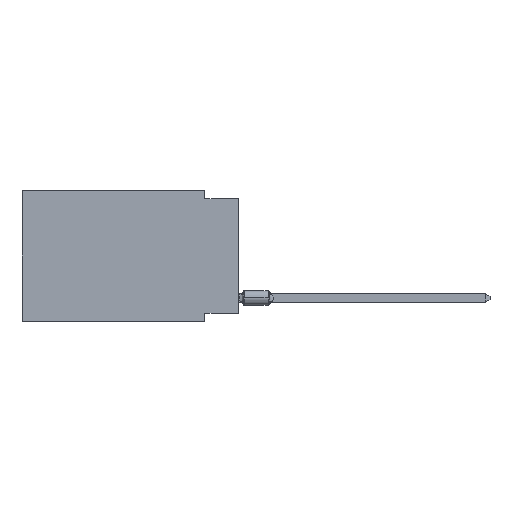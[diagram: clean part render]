
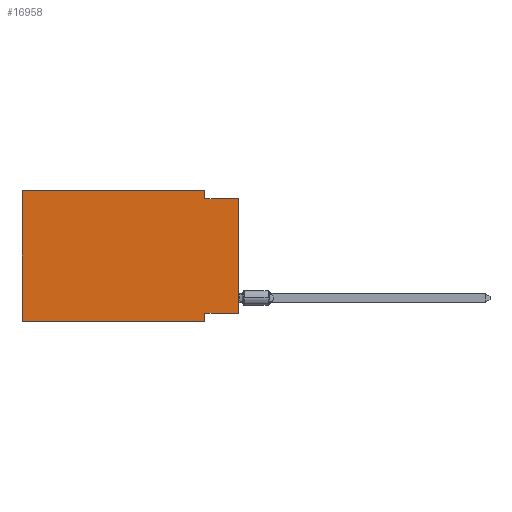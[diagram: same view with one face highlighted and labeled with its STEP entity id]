
A CAD part, left-side view. The second image highlights one B-rep face of the part: STEP entity #16958.
In plain terms, the highlighted planar face has unit normal (-1, 0, 0).
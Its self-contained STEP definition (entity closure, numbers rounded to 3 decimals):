
#176 = LINE ( 'NONE', #9296, #8704 ) ;
#828 = LINE ( 'NONE', #19215, #23121 ) ;
#2320 = CARTESIAN_POINT ( 'NONE',  ( 0., 0., -9.271 ) ) ;
#2956 = CARTESIAN_POINT ( 'NONE',  ( 0., 0., -0.635 ) ) ;
#3770 = ORIENTED_EDGE ( 'NONE', *, *, #13536, .F. ) ;
#3858 = VERTEX_POINT ( 'NONE', #8941 ) ;
#3895 = ORIENTED_EDGE ( 'NONE', *, *, #22134, .F. ) ;
#4241 = CARTESIAN_POINT ( 'NONE',  ( 0., 2.54, -9.271 ) ) ;
#4247 = LINE ( 'NONE', #11578, #9498 ) ;
#4365 = DIRECTION ( 'NONE',  ( 0., -1., 0. ) ) ;
#4725 = VECTOR ( 'NONE', #18708, 1000. ) ;
#4831 = VECTOR ( 'NONE', #16319, 1000. ) ;
#5357 = EDGE_CURVE ( 'NONE', #22866, #3858, #14634, .T. ) ;
#6028 = LINE ( 'NONE', #20197, #18203 ) ;
#6499 = VERTEX_POINT ( 'NONE', #16546 ) ;
#6930 = CARTESIAN_POINT ( 'NONE',  ( 0., 2.54, 0. ) ) ;
#8102 = VERTEX_POINT ( 'NONE', #2956 ) ;
#8444 = EDGE_CURVE ( 'NONE', #16184, #11323, #11120, .T. ) ;
#8605 = CARTESIAN_POINT ( 'NONE',  ( 0., 0., -9.271 ) ) ;
#8704 = VECTOR ( 'NONE', #14965, 1000. ) ;
#8795 = VERTEX_POINT ( 'NONE', #11437 ) ;
#8941 = CARTESIAN_POINT ( 'NONE',  ( 0., 2.54, -0.635 ) ) ;
#9033 = AXIS2_PLACEMENT_3D ( 'NONE', #9889, #17216, #15758 ) ;
#9296 = CARTESIAN_POINT ( 'NONE',  ( 0., 16.383, -9.906 ) ) ;
#9498 = VECTOR ( 'NONE', #4365, 1000. ) ;
#9889 = CARTESIAN_POINT ( 'NONE',  ( 0., 16.383, 0. ) ) ;
#10449 = ORIENTED_EDGE ( 'NONE', *, *, #5357, .F. ) ;
#11120 = LINE ( 'NONE', #2320, #17021 ) ;
#11298 = CARTESIAN_POINT ( 'NONE',  ( 0., 2.54, 0. ) ) ;
#11323 = VERTEX_POINT ( 'NONE', #4241 ) ;
#11437 = CARTESIAN_POINT ( 'NONE',  ( 0., 16.383, 0. ) ) ;
#11578 = CARTESIAN_POINT ( 'NONE',  ( 0., 0., -0.635 ) ) ;
#11959 = ORIENTED_EDGE ( 'NONE', *, *, #8444, .F. ) ;
#12789 = VERTEX_POINT ( 'NONE', #18444 ) ;
#13177 = CARTESIAN_POINT ( 'NONE',  ( 0., 16.383, 0. ) ) ;
#13220 = VECTOR ( 'NONE', #20702, 1000. ) ;
#13288 = DIRECTION ( 'NONE',  ( 0., 1., 0. ) ) ;
#13536 = EDGE_CURVE ( 'NONE', #8795, #22866, #18577, .T. ) ;
#13750 = PLANE ( 'NONE',  #9033 ) ;
#14634 = LINE ( 'NONE', #6930, #4831 ) ;
#14965 = DIRECTION ( 'NONE',  ( 0., -1., 0. ) ) ;
#15092 = EDGE_LOOP ( 'NONE', ( #20683, #3895, #10449, #3770, #20002, #21562, #21787, #11959 ) ) ;
#15757 = EDGE_CURVE ( 'NONE', #16184, #8102, #828, .T. ) ;
#15758 = DIRECTION ( 'NONE',  ( 0., 0., -1. ) ) ;
#16184 = VERTEX_POINT ( 'NONE', #8605 ) ;
#16319 = DIRECTION ( 'NONE',  ( 0., 0., -1. ) ) ;
#16546 = CARTESIAN_POINT ( 'NONE',  ( 0., 16.383, -9.906 ) ) ;
#16851 = DIRECTION ( 'NONE',  ( 0., 0., 1. ) ) ;
#16958 = ADVANCED_FACE ( 'NONE', ( #19009 ), #13750, .F. ) ;
#17021 = VECTOR ( 'NONE', #13288, 1000. ) ;
#17216 = DIRECTION ( 'NONE',  ( 1., 0., 0. ) ) ;
#18015 = EDGE_CURVE ( 'NONE', #11323, #12789, #19367, .T. ) ;
#18203 = VECTOR ( 'NONE', #16851, 1000. ) ;
#18444 = CARTESIAN_POINT ( 'NONE',  ( 0., 2.54, -9.906 ) ) ;
#18577 = LINE ( 'NONE', #13177, #4725 ) ;
#18708 = DIRECTION ( 'NONE',  ( 0., -1., 0. ) ) ;
#19009 = FACE_OUTER_BOUND ( 'NONE', #15092, .T. ) ;
#19215 = CARTESIAN_POINT ( 'NONE',  ( 0., 0., 0. ) ) ;
#19367 = LINE ( 'NONE', #20937, #13220 ) ;
#19552 = EDGE_CURVE ( 'NONE', #6499, #8795, #6028, .T. ) ;
#20002 = ORIENTED_EDGE ( 'NONE', *, *, #19552, .F. ) ;
#20197 = CARTESIAN_POINT ( 'NONE',  ( 0., 16.383, 0. ) ) ;
#20683 = ORIENTED_EDGE ( 'NONE', *, *, #15757, .T. ) ;
#20702 = DIRECTION ( 'NONE',  ( 0., 0., -1. ) ) ;
#20937 = CARTESIAN_POINT ( 'NONE',  ( 0., 2.54, -9.906 ) ) ;
#21562 = ORIENTED_EDGE ( 'NONE', *, *, #23695, .T. ) ;
#21787 = ORIENTED_EDGE ( 'NONE', *, *, #18015, .F. ) ;
#22134 = EDGE_CURVE ( 'NONE', #3858, #8102, #4247, .T. ) ;
#22866 = VERTEX_POINT ( 'NONE', #11298 ) ;
#23037 = DIRECTION ( 'NONE',  ( 0., 0., 1. ) ) ;
#23121 = VECTOR ( 'NONE', #23037, 1000. ) ;
#23695 = EDGE_CURVE ( 'NONE', #6499, #12789, #176, .T. ) ;
